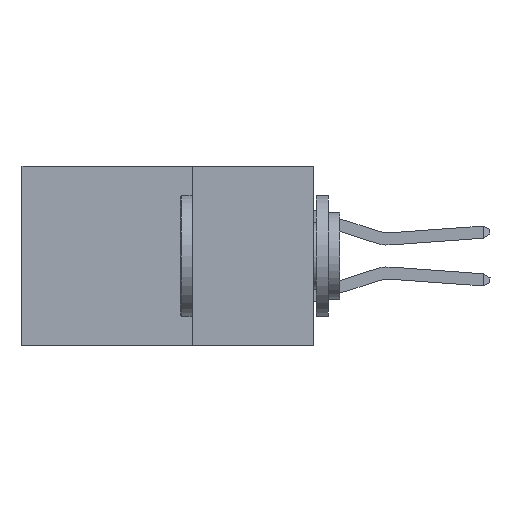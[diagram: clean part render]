
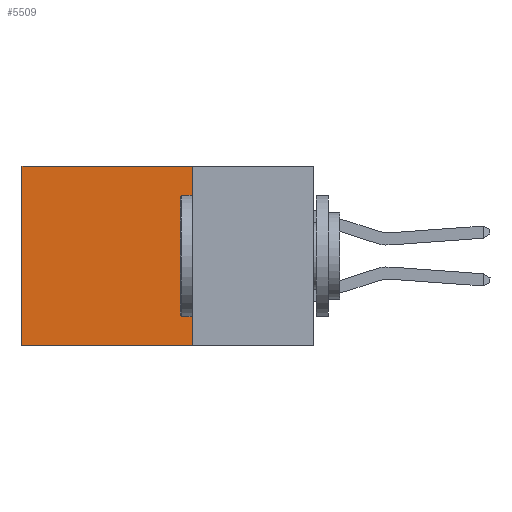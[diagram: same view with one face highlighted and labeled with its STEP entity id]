
A CAD part, left-side view. The second image highlights one B-rep face of the part: STEP entity #5509.
In plain terms, the highlighted planar face has unit normal (-1, 0, 0).
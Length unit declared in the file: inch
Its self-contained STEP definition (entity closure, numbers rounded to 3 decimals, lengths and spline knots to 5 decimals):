
#1408 = CARTESIAN_POINT ( 'NONE',  ( 0.2875, 0.25, 0. ) ) ;
#1568 = LINE ( 'NONE', #1408, #9647 ) ;
#1603 = DIRECTION ( 'NONE',  ( 0., 1., 0. ) ) ;
#1817 = FACE_OUTER_BOUND ( 'NONE', #12894, .T. ) ;
#2297 = ORIENTED_EDGE ( 'NONE', *, *, #4198, .T. ) ;
#3331 = ORIENTED_EDGE ( 'NONE', *, *, #10266, .F. ) ;
#3504 = CARTESIAN_POINT ( 'NONE',  ( 0.2875, 0.6, 0. ) ) ;
#3620 = PLANE ( 'NONE',  #16796 ) ;
#3898 = CARTESIAN_POINT ( 'NONE',  ( 0.2875, 0.25, -0.37 ) ) ;
#4090 = LINE ( 'NONE', #11182, #19348 ) ;
#4179 = VERTEX_POINT ( 'NONE', #17083 ) ;
#4198 = EDGE_CURVE ( 'NONE', #17836, #4179, #4090, .T. ) ;
#5509 = ADVANCED_FACE ( 'NONE', ( #1817 ), #3620, .F. ) ;
#6017 = CARTESIAN_POINT ( 'NONE',  ( 0.2875, 0.25, 0. ) ) ;
#6324 = EDGE_CURVE ( 'NONE', #17382, #10161, #1568, .T. ) ;
#6413 = EDGE_CURVE ( 'NONE', #17382, #17836, #11433, .T. ) ;
#6644 = DIRECTION ( 'NONE',  ( 0., 0., -1. ) ) ;
#7485 = VECTOR ( 'NONE', #1603, 39.37008 ) ;
#9647 = VECTOR ( 'NONE', #11955, 39.37008 ) ;
#10161 = VERTEX_POINT ( 'NONE', #11152 ) ;
#10266 = EDGE_CURVE ( 'NONE', #10161, #4179, #18438, .T. ) ;
#11099 = ORIENTED_EDGE ( 'NONE', *, *, #6413, .T. ) ;
#11152 = CARTESIAN_POINT ( 'NONE',  ( 0.2875, 0.25, -0.37 ) ) ;
#11182 = CARTESIAN_POINT ( 'NONE',  ( 0.2875, 0.6, 0. ) ) ;
#11433 = LINE ( 'NONE', #15077, #7485 ) ;
#11955 = DIRECTION ( 'NONE',  ( 0., 0., -1. ) ) ;
#12823 = ORIENTED_EDGE ( 'NONE', *, *, #6324, .F. ) ;
#12825 = DIRECTION ( 'NONE',  ( 0., 1., 0. ) ) ;
#12894 = EDGE_LOOP ( 'NONE', ( #2297, #3331, #12823, #11099 ) ) ;
#14051 = CARTESIAN_POINT ( 'NONE',  ( 0.2875, 0.25, 0. ) ) ;
#15077 = CARTESIAN_POINT ( 'NONE',  ( 0.2875, 0.25, 0. ) ) ;
#15549 = DIRECTION ( 'NONE',  ( 1., 0., 0. ) ) ;
#15657 = DIRECTION ( 'NONE',  ( 0., 0., -1. ) ) ;
#16796 = AXIS2_PLACEMENT_3D ( 'NONE', #14051, #15549, #6644 ) ;
#17083 = CARTESIAN_POINT ( 'NONE',  ( 0.2875, 0.6, -0.37 ) ) ;
#17382 = VERTEX_POINT ( 'NONE', #6017 ) ;
#17836 = VERTEX_POINT ( 'NONE', #3504 ) ;
#17987 = VECTOR ( 'NONE', #12825, 39.37008 ) ;
#18438 = LINE ( 'NONE', #3898, #17987 ) ;
#19348 = VECTOR ( 'NONE', #15657, 39.37008 ) ;
